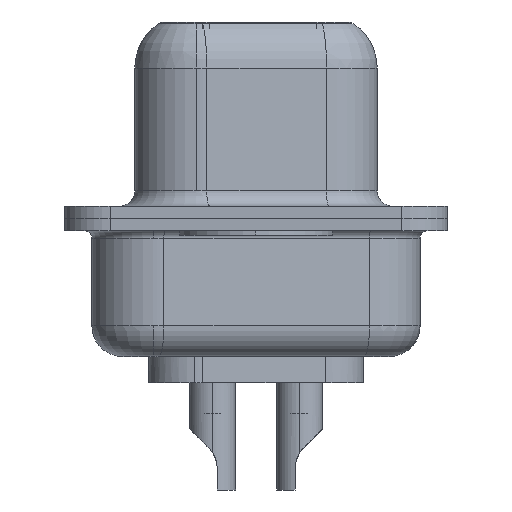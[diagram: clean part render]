
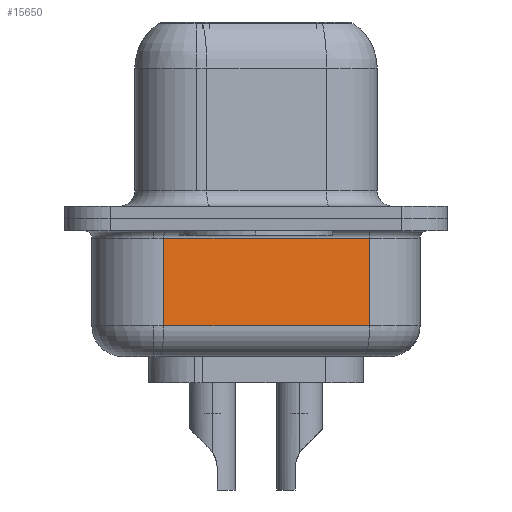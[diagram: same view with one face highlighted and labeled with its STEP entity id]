
A CAD part, left-side view. The second image highlights one B-rep face of the part: STEP entity #15650.
In plain terms, the highlighted planar face has unit normal (-0.985, -0.174, 0).
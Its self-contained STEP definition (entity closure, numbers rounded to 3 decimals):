
#465 = VECTOR ( 'NONE', #11800, 1000. ) ;
#1609 = DIRECTION ( 'NONE',  ( 0., 0., 1. ) ) ;
#1654 = VERTEX_POINT ( 'NONE', #2379 ) ;
#2379 = CARTESIAN_POINT ( 'NONE',  ( 4.062, -3.697, -0.65 ) ) ;
#3376 = CARTESIAN_POINT ( 'NONE',  ( 2.88, 3.003, -4.5 ) ) ;
#4730 = CARTESIAN_POINT ( 'NONE',  ( 2.88, 3.003, -4.5 ) ) ;
#5762 = ORIENTED_EDGE ( 'NONE', *, *, #10782, .T. ) ;
#5992 = CARTESIAN_POINT ( 'NONE',  ( 2.88, 3.003, -0.65 ) ) ;
#6627 = PLANE ( 'NONE',  #13091 ) ;
#7794 = DIRECTION ( 'NONE',  ( 0.174, -0.985, 0. ) ) ;
#8118 = VECTOR ( 'NONE', #1609, 1000. ) ;
#9138 = EDGE_CURVE ( 'NONE', #15287, #19870, #19498, .T. ) ;
#9418 = DIRECTION ( 'NONE',  ( 0., 0., 1. ) ) ;
#9757 = LINE ( 'NONE', #5992, #465 ) ;
#10389 = VERTEX_POINT ( 'NONE', #17272 ) ;
#10392 = DIRECTION ( 'NONE',  ( -0.174, 0.985, 0. ) ) ;
#10782 = EDGE_CURVE ( 'NONE', #1654, #10389, #9757, .T. ) ;
#10805 = CARTESIAN_POINT ( 'NONE',  ( 4.062, -3.697, -4.5 ) ) ;
#11800 = DIRECTION ( 'NONE',  ( -0.174, 0.985, 0. ) ) ;
#13091 = AXIS2_PLACEMENT_3D ( 'NONE', #4730, #22094, #10392 ) ;
#13703 = EDGE_CURVE ( 'NONE', #15287, #10389, #22754, .T. ) ;
#14850 = VECTOR ( 'NONE', #7794, 1000. ) ;
#15287 = VERTEX_POINT ( 'NONE', #23886 ) ;
#15650 = ADVANCED_FACE ( 'NONE', ( #20089 ), #6627, .F. ) ;
#15785 = ORIENTED_EDGE ( 'NONE', *, *, #19097, .T. ) ;
#16564 = CARTESIAN_POINT ( 'NONE',  ( 4.062, -3.697, -3.5 ) ) ;
#17051 = VECTOR ( 'NONE', #9418, 1000. ) ;
#17062 = ORIENTED_EDGE ( 'NONE', *, *, #13703, .F. ) ;
#17272 = CARTESIAN_POINT ( 'NONE',  ( 2.88, 3.003, -0.65 ) ) ;
#17746 = ORIENTED_EDGE ( 'NONE', *, *, #9138, .T. ) ;
#19097 = EDGE_CURVE ( 'NONE', #19870, #1654, #22619, .T. ) ;
#19498 = LINE ( 'NONE', #19613, #14850 ) ;
#19613 = CARTESIAN_POINT ( 'NONE',  ( 2.88, 3.003, -3.5 ) ) ;
#19870 = VERTEX_POINT ( 'NONE', #16564 ) ;
#20089 = FACE_OUTER_BOUND ( 'NONE', #21163, .T. ) ;
#21163 = EDGE_LOOP ( 'NONE', ( #17062, #17746, #15785, #5762 ) ) ;
#22094 = DIRECTION ( 'NONE',  ( 0.985, 0.174, 0. ) ) ;
#22619 = LINE ( 'NONE', #10805, #8118 ) ;
#22754 = LINE ( 'NONE', #3376, #17051 ) ;
#23886 = CARTESIAN_POINT ( 'NONE',  ( 2.88, 3.003, -3.5 ) ) ;
